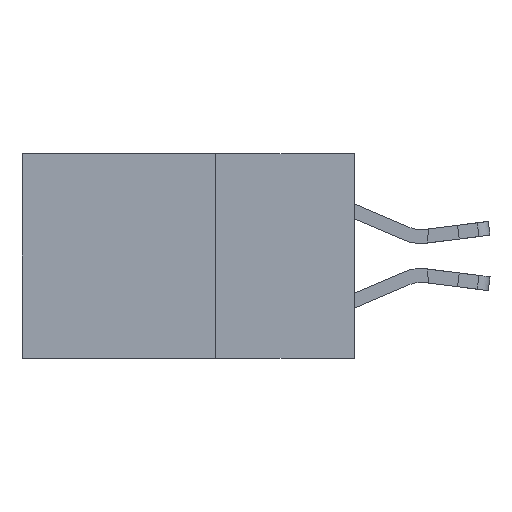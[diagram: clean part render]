
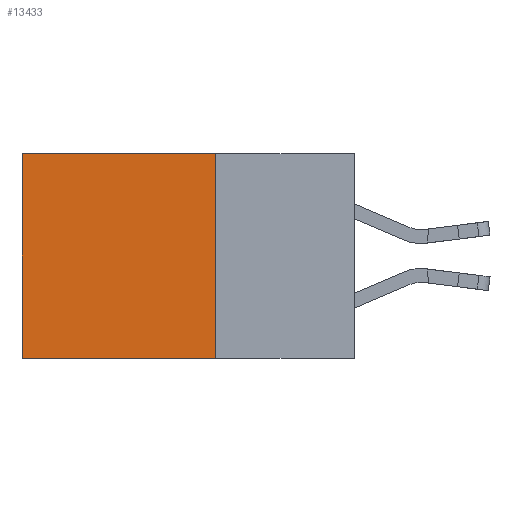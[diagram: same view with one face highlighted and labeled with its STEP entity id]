
A CAD part, left-side view. The second image highlights one B-rep face of the part: STEP entity #13433.
In plain terms, the highlighted planar face has unit normal (-1, 0, 0).
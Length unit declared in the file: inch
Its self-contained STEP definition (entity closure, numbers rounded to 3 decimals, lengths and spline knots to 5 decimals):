
#3 = AXIS2_PLACEMENT_3D ( 'NONE', #16150, #18030, #6727 ) ;
#1434 = LINE ( 'NONE', #4286, #14781 ) ;
#2037 = ORIENTED_EDGE ( 'NONE', *, *, #9378, .T. ) ;
#4286 = CARTESIAN_POINT ( 'NONE',  ( 0.298, 0.25, 0. ) ) ;
#4918 = VECTOR ( 'NONE', #5635, 39.37008 ) ;
#5635 = DIRECTION ( 'NONE',  ( 0., 1., 0. ) ) ;
#5748 = CARTESIAN_POINT ( 'NONE',  ( 0.298, 0.25, 0. ) ) ;
#6650 = VERTEX_POINT ( 'NONE', #10085 ) ;
#6727 = DIRECTION ( 'NONE',  ( 0., 0., -1. ) ) ;
#7198 = ORIENTED_EDGE ( 'NONE', *, *, #7592, .F. ) ;
#7486 = CARTESIAN_POINT ( 'NONE',  ( 0.298, 0.6, 0. ) ) ;
#7592 = EDGE_CURVE ( 'NONE', #14962, #6650, #8776, .T. ) ;
#7745 = DIRECTION ( 'NONE',  ( 0., 1., 0. ) ) ;
#8776 = LINE ( 'NONE', #22515, #4918 ) ;
#9378 = EDGE_CURVE ( 'NONE', #10095, #9961, #16688, .T. ) ;
#9961 = VERTEX_POINT ( 'NONE', #7486 ) ;
#9971 = DIRECTION ( 'NONE',  ( 0., 0., -1. ) ) ;
#10085 = CARTESIAN_POINT ( 'NONE',  ( 0.298, 0.6, -0.37 ) ) ;
#10095 = VERTEX_POINT ( 'NONE', #5748 ) ;
#11526 = CARTESIAN_POINT ( 'NONE',  ( 0.298, 0.6, 0. ) ) ;
#11820 = EDGE_CURVE ( 'NONE', #10095, #14962, #1434, .T. ) ;
#13433 = ADVANCED_FACE ( 'NONE', ( #23229 ), #23980, .F. ) ;
#14638 = ORIENTED_EDGE ( 'NONE', *, *, #11820, .F. ) ;
#14781 = VECTOR ( 'NONE', #23175, 39.37008 ) ;
#14902 = EDGE_LOOP ( 'NONE', ( #19609, #7198, #14638, #2037 ) ) ;
#14962 = VERTEX_POINT ( 'NONE', #15224 ) ;
#15224 = CARTESIAN_POINT ( 'NONE',  ( 0.298, 0.25, -0.37 ) ) ;
#15460 = LINE ( 'NONE', #11526, #16956 ) ;
#16150 = CARTESIAN_POINT ( 'NONE',  ( 0.298, 0.25, 0. ) ) ;
#16688 = LINE ( 'NONE', #24516, #23144 ) ;
#16956 = VECTOR ( 'NONE', #9971, 39.37008 ) ;
#17603 = EDGE_CURVE ( 'NONE', #9961, #6650, #15460, .T. ) ;
#18030 = DIRECTION ( 'NONE',  ( 1., 0., 0. ) ) ;
#19609 = ORIENTED_EDGE ( 'NONE', *, *, #17603, .T. ) ;
#22515 = CARTESIAN_POINT ( 'NONE',  ( 0.298, 0.25, -0.37 ) ) ;
#23144 = VECTOR ( 'NONE', #7745, 39.37008 ) ;
#23175 = DIRECTION ( 'NONE',  ( 0., 0., -1. ) ) ;
#23229 = FACE_OUTER_BOUND ( 'NONE', #14902, .T. ) ;
#23980 = PLANE ( 'NONE',  #3 ) ;
#24516 = CARTESIAN_POINT ( 'NONE',  ( 0.298, 0.25, 0. ) ) ;
